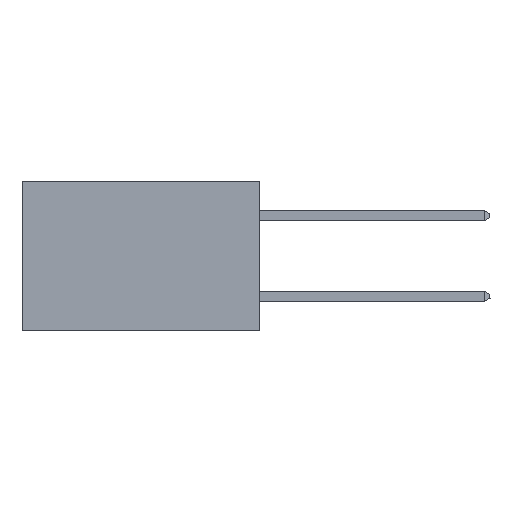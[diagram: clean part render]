
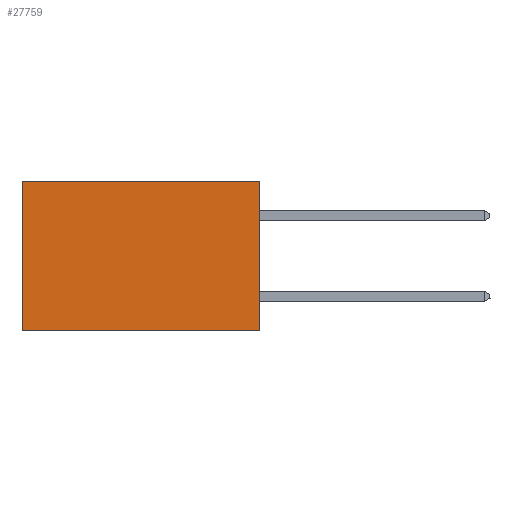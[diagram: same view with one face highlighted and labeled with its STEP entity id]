
A CAD part, left-side view. The second image highlights one B-rep face of the part: STEP entity #27759.
In plain terms, the highlighted planar face has unit normal (-1, 0, 0).
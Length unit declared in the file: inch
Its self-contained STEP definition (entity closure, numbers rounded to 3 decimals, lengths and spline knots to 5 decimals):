
#1247 = ORIENTED_EDGE ( 'NONE', *, *, #10601, .F. ) ;
#2240 = PLANE ( 'NONE',  #27357 ) ;
#2343 = EDGE_CURVE ( 'NONE', #25764, #17153, #18916, .T. ) ;
#3015 = ORIENTED_EDGE ( 'NONE', *, *, #12827, .T. ) ;
#3446 = CARTESIAN_POINT ( 'NONE',  ( 0.277, 0., -0.37 ) ) ;
#3789 = DIRECTION ( 'NONE',  ( 0., 0., -1. ) ) ;
#4280 = CARTESIAN_POINT ( 'NONE',  ( 0.277, 0., -0.37 ) ) ;
#4552 = CARTESIAN_POINT ( 'NONE',  ( 0.277, 0., -0.37 ) ) ;
#4946 = ORIENTED_EDGE ( 'NONE', *, *, #10389, .T. ) ;
#5230 = FACE_OUTER_BOUND ( 'NONE', #15204, .T. ) ;
#6096 = CARTESIAN_POINT ( 'NONE',  ( 0.277, 0.59, -0.37 ) ) ;
#6135 = VECTOR ( 'NONE', #3789, 39.37008 ) ;
#6913 = DIRECTION ( 'NONE',  ( 0., 0., -1. ) ) ;
#7048 = VECTOR ( 'NONE', #28657, 39.37008 ) ;
#8093 = CARTESIAN_POINT ( 'NONE',  ( 0.277, 0.59, 0. ) ) ;
#10389 = EDGE_CURVE ( 'NONE', #25764, #12000, #24379, .T. ) ;
#10601 = EDGE_CURVE ( 'NONE', #17153, #28929, #19297, .T. ) ;
#12000 = VERTEX_POINT ( 'NONE', #8093 ) ;
#12019 = CARTESIAN_POINT ( 'NONE',  ( 0.277, 0., 0. ) ) ;
#12811 = VECTOR ( 'NONE', #14349, 39.37008 ) ;
#12827 = EDGE_CURVE ( 'NONE', #12000, #28929, #24588, .T. ) ;
#14349 = DIRECTION ( 'NONE',  ( 0., 1., 0. ) ) ;
#15204 = EDGE_LOOP ( 'NONE', ( #3015, #1247, #28943, #4946 ) ) ;
#17153 = VERTEX_POINT ( 'NONE', #4280 ) ;
#18916 = LINE ( 'NONE', #23726, #24353 ) ;
#19297 = LINE ( 'NONE', #3446, #7048 ) ;
#19517 = CARTESIAN_POINT ( 'NONE',  ( 0.277, 0.59, -0.37 ) ) ;
#20757 = DIRECTION ( 'NONE',  ( 1., 0., 0. ) ) ;
#21070 = CARTESIAN_POINT ( 'NONE',  ( 0.277, 0., 0. ) ) ;
#23726 = CARTESIAN_POINT ( 'NONE',  ( 0.277, 0., -0.37 ) ) ;
#24353 = VECTOR ( 'NONE', #24462, 39.37008 ) ;
#24379 = LINE ( 'NONE', #12019, #12811 ) ;
#24462 = DIRECTION ( 'NONE',  ( 0., 0., -1. ) ) ;
#24588 = LINE ( 'NONE', #6096, #6135 ) ;
#25764 = VERTEX_POINT ( 'NONE', #21070 ) ;
#27357 = AXIS2_PLACEMENT_3D ( 'NONE', #4552, #20757, #6913 ) ;
#27759 = ADVANCED_FACE ( 'NONE', ( #5230 ), #2240, .F. ) ;
#28657 = DIRECTION ( 'NONE',  ( 0., 1., 0. ) ) ;
#28929 = VERTEX_POINT ( 'NONE', #19517 ) ;
#28943 = ORIENTED_EDGE ( 'NONE', *, *, #2343, .F. ) ;
